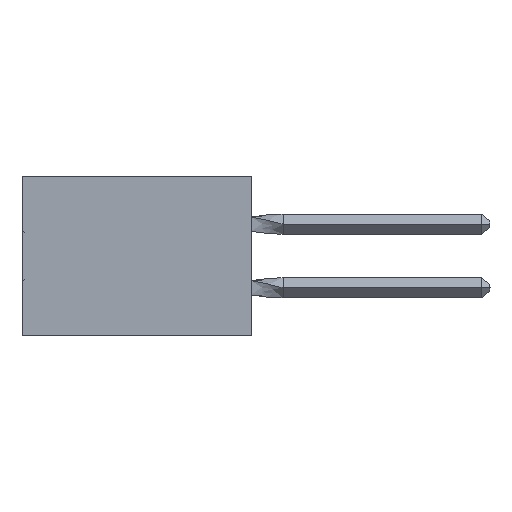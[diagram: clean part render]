
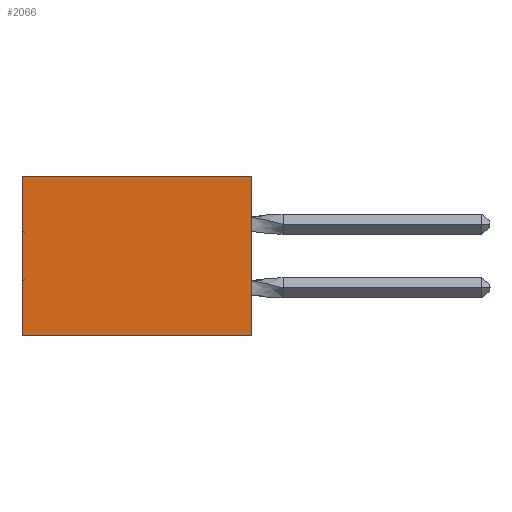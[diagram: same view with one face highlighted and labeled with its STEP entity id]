
A CAD part, left-side view. The second image highlights one B-rep face of the part: STEP entity #2066.
In plain terms, the highlighted planar face has unit normal (-1, 0, 0).
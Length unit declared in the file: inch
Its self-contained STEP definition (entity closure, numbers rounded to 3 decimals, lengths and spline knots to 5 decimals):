
#401 = EDGE_CURVE ( 'NONE', #21038, #3485, #18999, .T. ) ;
#637 = EDGE_CURVE ( 'NONE', #21038, #50171, #7355, .T. ) ;
#647 = VECTOR ( 'NONE', #41090, 39.37008 ) ;
#2066 = ADVANCED_FACE ( 'NONE', ( #3241 ), #40895, .F. ) ;
#3241 = FACE_OUTER_BOUND ( 'NONE', #55300, .T. ) ;
#3485 = VERTEX_POINT ( 'NONE', #35185 ) ;
#7355 = LINE ( 'NONE', #10686, #647 ) ;
#8725 = VERTEX_POINT ( 'NONE', #23724 ) ;
#10092 = DIRECTION ( 'NONE',  ( 0., 1., 0. ) ) ;
#10686 = CARTESIAN_POINT ( 'NONE',  ( 0.305, 0., -0.5 ) ) ;
#12102 = ORIENTED_EDGE ( 'NONE', *, *, #401, .T. ) ;
#12985 = ORIENTED_EDGE ( 'NONE', *, *, #17042, .F. ) ;
#15034 = CARTESIAN_POINT ( 'NONE',  ( 0.305, 0., -0.5 ) ) ;
#15460 = CARTESIAN_POINT ( 'NONE',  ( 0.305, 0.72, -0.5 ) ) ;
#17042 = EDGE_CURVE ( 'NONE', #50171, #8725, #52946, .T. ) ;
#18999 = LINE ( 'NONE', #46565, #40115 ) ;
#19471 = LINE ( 'NONE', #15460, #45352 ) ;
#21038 = VERTEX_POINT ( 'NONE', #37936 ) ;
#23040 = DIRECTION ( 'NONE',  ( 1., 0., 0. ) ) ;
#23724 = CARTESIAN_POINT ( 'NONE',  ( 0.305, 0.72, -0.5 ) ) ;
#27644 = DIRECTION ( 'NONE',  ( 0., 0., -1. ) ) ;
#28984 = DIRECTION ( 'NONE',  ( 0., 0., -1. ) ) ;
#29977 = EDGE_CURVE ( 'NONE', #3485, #8725, #19471, .T. ) ;
#35185 = CARTESIAN_POINT ( 'NONE',  ( 0.305, 0.72, 0. ) ) ;
#36765 = ORIENTED_EDGE ( 'NONE', *, *, #29977, .T. ) ;
#37936 = CARTESIAN_POINT ( 'NONE',  ( 0.305, 0., 0. ) ) ;
#38312 = DIRECTION ( 'NONE',  ( 0., 1., 0. ) ) ;
#39637 = CARTESIAN_POINT ( 'NONE',  ( 0.305, 0., -0.5 ) ) ;
#40115 = VECTOR ( 'NONE', #38312, 39.37008 ) ;
#40895 = PLANE ( 'NONE',  #52079 ) ;
#41090 = DIRECTION ( 'NONE',  ( 0., 0., -1. ) ) ;
#42035 = VECTOR ( 'NONE', #10092, 39.37008 ) ;
#42244 = ORIENTED_EDGE ( 'NONE', *, *, #637, .F. ) ;
#45352 = VECTOR ( 'NONE', #28984, 39.37008 ) ;
#46565 = CARTESIAN_POINT ( 'NONE',  ( 0.305, 0., 0. ) ) ;
#49865 = CARTESIAN_POINT ( 'NONE',  ( 0.305, 0., -0.5 ) ) ;
#50171 = VERTEX_POINT ( 'NONE', #39637 ) ;
#52079 = AXIS2_PLACEMENT_3D ( 'NONE', #15034, #23040, #27644 ) ;
#52946 = LINE ( 'NONE', #49865, #42035 ) ;
#55300 = EDGE_LOOP ( 'NONE', ( #36765, #12985, #42244, #12102 ) ) ;
